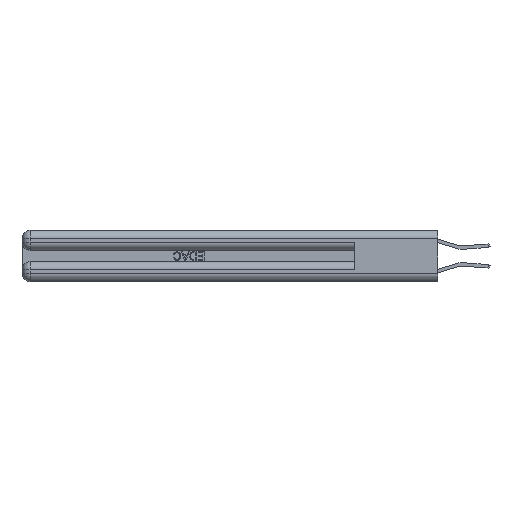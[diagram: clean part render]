
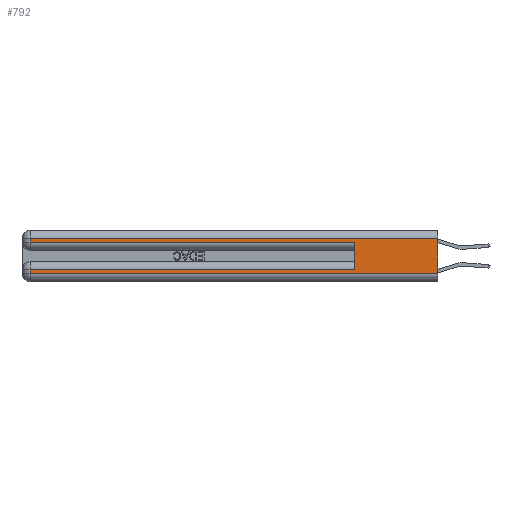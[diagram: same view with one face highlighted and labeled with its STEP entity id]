
A CAD part, left-side view. The second image highlights one B-rep face of the part: STEP entity #792.
In plain terms, the highlighted planar face has unit normal (-1, 0, 0).
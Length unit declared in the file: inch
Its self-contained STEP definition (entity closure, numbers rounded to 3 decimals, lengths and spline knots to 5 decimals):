
#170 = DIRECTION ( 'NONE',  ( 0., 0., -1. ) ) ;
#792 = ADVANCED_FACE ( 'NONE', ( #8152 ), #18413, .F. ) ;
#1376 = CARTESIAN_POINT ( 'NONE',  ( 0., 0., 0.06 ) ) ;
#2226 = CARTESIAN_POINT ( 'NONE',  ( 0., 0.6, 0.285 ) ) ;
#2285 = VERTEX_POINT ( 'NONE', #32361 ) ;
#2614 = EDGE_CURVE ( 'NONE', #20125, #33290, #21258, .T. ) ;
#3068 = VERTEX_POINT ( 'NONE', #20367 ) ;
#3332 = LINE ( 'NONE', #17535, #6104 ) ;
#4243 = ORIENTED_EDGE ( 'NONE', *, *, #20453, .T. ) ;
#4510 = EDGE_CURVE ( 'NONE', #32410, #3068, #11189, .T. ) ;
#5239 = EDGE_CURVE ( 'NONE', #3068, #11222, #21435, .T. ) ;
#6104 = VECTOR ( 'NONE', #17715, 39.37008 ) ;
#6180 = LINE ( 'NONE', #30915, #10797 ) ;
#6218 = CARTESIAN_POINT ( 'NONE',  ( 0., 0.6, 0.085 ) ) ;
#6761 = VECTOR ( 'NONE', #12988, 39.37008 ) ;
#7614 = LINE ( 'NONE', #23377, #6761 ) ;
#8152 = FACE_OUTER_BOUND ( 'NONE', #26952, .T. ) ;
#8331 = VECTOR ( 'NONE', #13118, 39.37008 ) ;
#9553 = VECTOR ( 'NONE', #170, 39.37008 ) ;
#10253 = DIRECTION ( 'NONE',  ( 1., 0., 0. ) ) ;
#10474 = VECTOR ( 'NONE', #19562, 39.37008 ) ;
#10480 = ORIENTED_EDGE ( 'NONE', *, *, #5239, .T. ) ;
#10797 = VECTOR ( 'NONE', #15155, 39.37008 ) ;
#10887 = CARTESIAN_POINT ( 'NONE',  ( 0., 2.94, 0.37 ) ) ;
#11189 = LINE ( 'NONE', #29171, #28835 ) ;
#11222 = VERTEX_POINT ( 'NONE', #23976 ) ;
#12988 = DIRECTION ( 'NONE',  ( 0., 0., -1. ) ) ;
#13118 = DIRECTION ( 'NONE',  ( 0., 1., 0. ) ) ;
#13825 = ORIENTED_EDGE ( 'NONE', *, *, #27906, .T. ) ;
#15155 = DIRECTION ( 'NONE',  ( 0., -1., 0. ) ) ;
#15268 = DIRECTION ( 'NONE',  ( 0., 0., -1. ) ) ;
#15416 = EDGE_CURVE ( 'NONE', #32410, #30411, #22475, .T. ) ;
#15447 = EDGE_CURVE ( 'NONE', #11222, #18351, #21799, .T. ) ;
#15524 = ORIENTED_EDGE ( 'NONE', *, *, #2614, .T. ) ;
#16357 = DIRECTION ( 'NONE',  ( 0., 1., 0. ) ) ;
#16531 = ORIENTED_EDGE ( 'NONE', *, *, #15447, .T. ) ;
#17371 = CARTESIAN_POINT ( 'NONE',  ( 0., 2.94, 0.31 ) ) ;
#17535 = CARTESIAN_POINT ( 'NONE',  ( 0., 2.94, 0.37 ) ) ;
#17715 = DIRECTION ( 'NONE',  ( 0., 0., -1. ) ) ;
#18351 = VERTEX_POINT ( 'NONE', #32021 ) ;
#18413 = PLANE ( 'NONE',  #28699 ) ;
#18508 = CARTESIAN_POINT ( 'NONE',  ( 0., 0., 0.31 ) ) ;
#19562 = DIRECTION ( 'NONE',  ( 0., 0., 1. ) ) ;
#20125 = VERTEX_POINT ( 'NONE', #33035 ) ;
#20367 = CARTESIAN_POINT ( 'NONE',  ( 0., 2.94, 0.085 ) ) ;
#20453 = EDGE_CURVE ( 'NONE', #2285, #30411, #6180, .T. ) ;
#21258 = LINE ( 'NONE', #18508, #8331 ) ;
#21435 = LINE ( 'NONE', #10887, #9553 ) ;
#21799 = LINE ( 'NONE', #1376, #23729 ) ;
#22475 = LINE ( 'NONE', #27159, #10474 ) ;
#22536 = ORIENTED_EDGE ( 'NONE', *, *, #29952, .F. ) ;
#23377 = CARTESIAN_POINT ( 'NONE',  ( 0., 0., 0.37 ) ) ;
#23486 = ORIENTED_EDGE ( 'NONE', *, *, #4510, .T. ) ;
#23729 = VECTOR ( 'NONE', #27683, 39.37008 ) ;
#23976 = CARTESIAN_POINT ( 'NONE',  ( 0., 2.94, 0.06 ) ) ;
#26952 = EDGE_LOOP ( 'NONE', ( #22536, #15524, #13825, #4243, #31048, #23486, #10480, #16531 ) ) ;
#27159 = CARTESIAN_POINT ( 'NONE',  ( 0., 0.6, 0.145 ) ) ;
#27683 = DIRECTION ( 'NONE',  ( 0., -1., 0. ) ) ;
#27906 = EDGE_CURVE ( 'NONE', #33290, #2285, #3332, .T. ) ;
#28699 = AXIS2_PLACEMENT_3D ( 'NONE', #34139, #10253, #15268 ) ;
#28835 = VECTOR ( 'NONE', #16357, 39.37008 ) ;
#29171 = CARTESIAN_POINT ( 'NONE',  ( 0., 0., 0.085 ) ) ;
#29952 = EDGE_CURVE ( 'NONE', #20125, #18351, #7614, .T. ) ;
#30411 = VERTEX_POINT ( 'NONE', #2226 ) ;
#30915 = CARTESIAN_POINT ( 'NONE',  ( 0., 0., 0.285 ) ) ;
#31048 = ORIENTED_EDGE ( 'NONE', *, *, #15416, .F. ) ;
#32021 = CARTESIAN_POINT ( 'NONE',  ( 0., 0., 0.06 ) ) ;
#32361 = CARTESIAN_POINT ( 'NONE',  ( 0., 2.94, 0.285 ) ) ;
#32410 = VERTEX_POINT ( 'NONE', #6218 ) ;
#33035 = CARTESIAN_POINT ( 'NONE',  ( 0., 0., 0.31 ) ) ;
#33290 = VERTEX_POINT ( 'NONE', #17371 ) ;
#34139 = CARTESIAN_POINT ( 'NONE',  ( 0., 0., 0.37 ) ) ;
